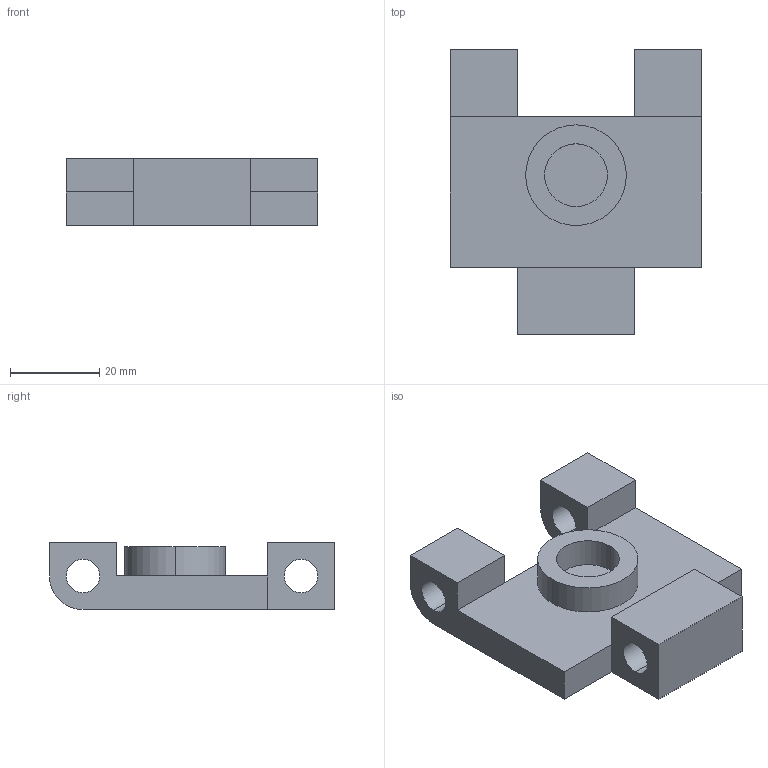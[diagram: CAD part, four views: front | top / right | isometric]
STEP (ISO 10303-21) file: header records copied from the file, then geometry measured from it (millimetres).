
FILE_DESCRIPTION (( 'STEP AP203' ), '1' );
FILE_NAME ('Back_Plate.STEP', '2013-09-22T12:16:09', ( '' ), ( '' ), 'SwSTEP 2.0', 'SolidWorks 2013', '' );
FILE_SCHEMA (( 'CONFIG_CONTROL_DESIGN' ));
Length unit declared in the file: millimetre
Products named in the file (1): Back_Plate
Bounding box: 56.25 x 63.75 x 15 mm (x, y, z)
Volume: 25639.8 mm3; surface area: 10697.4 mm2
Topology: 1 solids, 1 shells, 34 faces, 86 edges, 56 vertices
Faces by surface type: plane 22, cylinder 12
Entity records: 1111 total; most frequent: DIRECTION 180, CARTESIAN_POINT 177, ORIENTED_EDGE 172, EDGE_CURVE 86, VECTOR 62, LINE 62, AXIS2_PLACEMENT_3D 59, VERTEX_POINT 56
